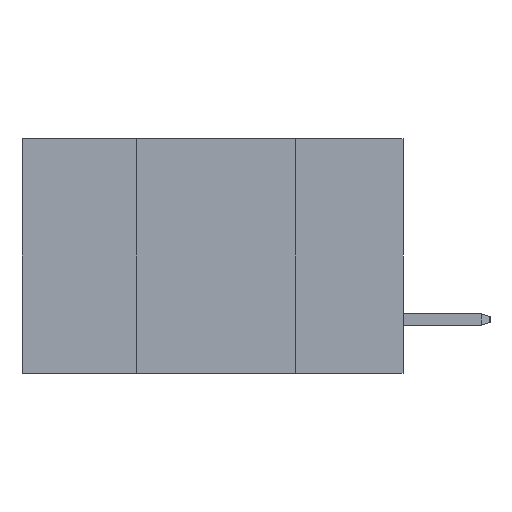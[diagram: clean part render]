
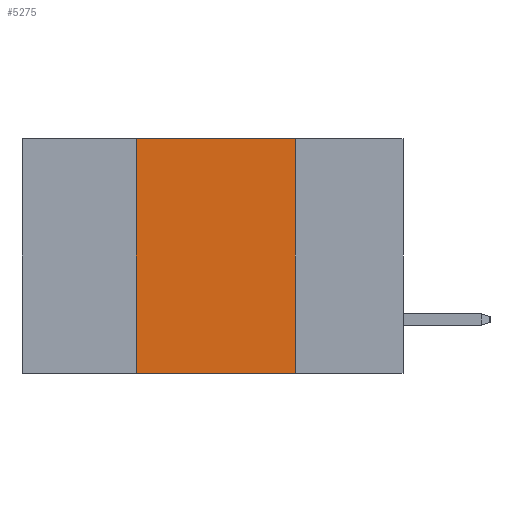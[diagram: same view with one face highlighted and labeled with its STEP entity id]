
A CAD part, left-side view. The second image highlights one B-rep face of the part: STEP entity #5275.
In plain terms, the highlighted planar face has unit normal (-1, 0, 0).
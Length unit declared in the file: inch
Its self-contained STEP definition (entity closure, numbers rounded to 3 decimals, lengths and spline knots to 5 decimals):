
#485 = EDGE_CURVE ( 'NONE', #5758, #2896, #12972, .T. ) ;
#1015 = PLANE ( 'NONE',  #8446 ) ;
#1385 = DIRECTION ( 'NONE',  ( 0., -1., 0. ) ) ;
#1680 = CARTESIAN_POINT ( 'NONE',  ( 0., 0.17, 0. ) ) ;
#2054 = DIRECTION ( 'NONE',  ( 0., -1., 0. ) ) ;
#2470 = ORIENTED_EDGE ( 'NONE', *, *, #485, .F. ) ;
#2845 = CARTESIAN_POINT ( 'NONE',  ( 0., 0.42, 0. ) ) ;
#2896 = VERTEX_POINT ( 'NONE', #1680 ) ;
#3152 = CARTESIAN_POINT ( 'NONE',  ( 0., 0.6, 0. ) ) ;
#3238 = VERTEX_POINT ( 'NONE', #12313 ) ;
#5041 = VERTEX_POINT ( 'NONE', #11875 ) ;
#5275 = ADVANCED_FACE ( 'NONE', ( #14407 ), #1015, .F. ) ;
#5758 = VERTEX_POINT ( 'NONE', #10720 ) ;
#6055 = ORIENTED_EDGE ( 'NONE', *, *, #9248, .F. ) ;
#7157 = VECTOR ( 'NONE', #12344, 39.37008 ) ;
#7314 = EDGE_LOOP ( 'NONE', ( #8432, #2470, #6055, #13808 ) ) ;
#7324 = LINE ( 'NONE', #14700, #9773 ) ;
#8432 = ORIENTED_EDGE ( 'NONE', *, *, #9234, .F. ) ;
#8446 = AXIS2_PLACEMENT_3D ( 'NONE', #9278, #9509, #9356 ) ;
#8821 = CARTESIAN_POINT ( 'NONE',  ( 0., 0.17, 0. ) ) ;
#9234 = EDGE_CURVE ( 'NONE', #2896, #3238, #11386, .T. ) ;
#9248 = EDGE_CURVE ( 'NONE', #5041, #5758, #14744, .T. ) ;
#9278 = CARTESIAN_POINT ( 'NONE',  ( 0., 0.6, 0. ) ) ;
#9356 = DIRECTION ( 'NONE',  ( 0., 0., -1. ) ) ;
#9509 = DIRECTION ( 'NONE',  ( 1., 0., 0. ) ) ;
#9773 = VECTOR ( 'NONE', #1385, 39.37008 ) ;
#10720 = CARTESIAN_POINT ( 'NONE',  ( 0., 0.42, 0. ) ) ;
#11386 = LINE ( 'NONE', #8821, #13312 ) ;
#11875 = CARTESIAN_POINT ( 'NONE',  ( 0., 0.42, -0.37 ) ) ;
#12313 = CARTESIAN_POINT ( 'NONE',  ( 0., 0.17, -0.37 ) ) ;
#12344 = DIRECTION ( 'NONE',  ( 0., 0., 1. ) ) ;
#12436 = DIRECTION ( 'NONE',  ( 0., 0., -1. ) ) ;
#12548 = EDGE_CURVE ( 'NONE', #5041, #3238, #7324, .T. ) ;
#12972 = LINE ( 'NONE', #3152, #14939 ) ;
#13312 = VECTOR ( 'NONE', #12436, 39.37008 ) ;
#13808 = ORIENTED_EDGE ( 'NONE', *, *, #12548, .T. ) ;
#14407 = FACE_OUTER_BOUND ( 'NONE', #7314, .T. ) ;
#14700 = CARTESIAN_POINT ( 'NONE',  ( 0., 0.6, -0.37 ) ) ;
#14744 = LINE ( 'NONE', #2845, #7157 ) ;
#14939 = VECTOR ( 'NONE', #2054, 39.37008 ) ;
